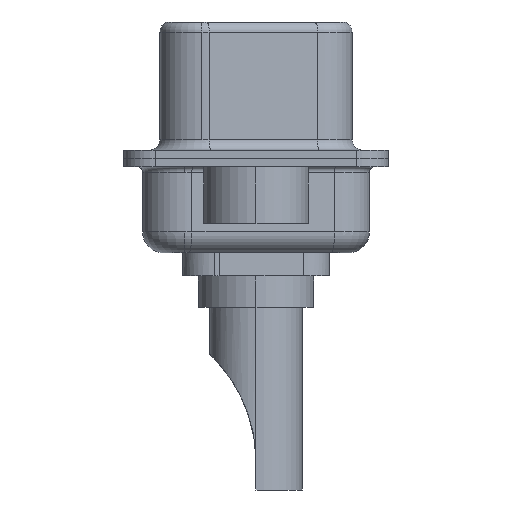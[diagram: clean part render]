
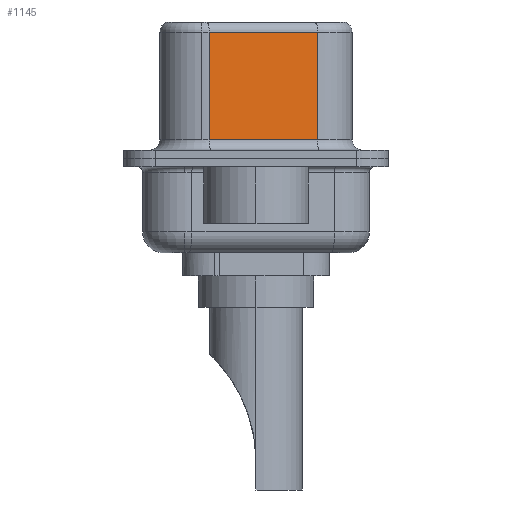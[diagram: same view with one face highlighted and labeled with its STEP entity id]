
A CAD part, left-side view. The second image highlights one B-rep face of the part: STEP entity #1145.
In plain terms, the highlighted planar face has unit normal (-0.985, -0.174, 0).
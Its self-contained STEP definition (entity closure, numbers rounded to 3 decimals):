
#921 = ORIENTED_EDGE ( 'NONE', *, *, #18159, .F. ) ;
#1145 = ADVANCED_FACE ( 'NONE', ( #7313 ), #12978, .F. ) ;
#1461 = CARTESIAN_POINT ( 'NONE',  ( 4.585, -2.927, 0.9 ) ) ;
#3293 = VERTEX_POINT ( 'NONE', #5164 ) ;
#3413 = VERTEX_POINT ( 'NONE', #20623 ) ;
#5068 = LINE ( 'NONE', #6559, #18393 ) ;
#5164 = CARTESIAN_POINT ( 'NONE',  ( 3.675, 2.233, 6.02 ) ) ;
#5823 = ORIENTED_EDGE ( 'NONE', *, *, #14037, .T. ) ;
#6559 = CARTESIAN_POINT ( 'NONE',  ( 4.585, -2.927, 0.9 ) ) ;
#7313 = FACE_OUTER_BOUND ( 'NONE', #21106, .T. ) ;
#7506 = DIRECTION ( 'NONE',  ( -0.174, 0.985, 0. ) ) ;
#8138 = VECTOR ( 'NONE', #14675, 1000. ) ;
#8716 = VECTOR ( 'NONE', #13194, 1000. ) ;
#10088 = ORIENTED_EDGE ( 'NONE', *, *, #10400, .T. ) ;
#10400 = EDGE_CURVE ( 'NONE', #3293, #3413, #13261, .T. ) ;
#10578 = ORIENTED_EDGE ( 'NONE', *, *, #11546, .T. ) ;
#11383 = CARTESIAN_POINT ( 'NONE',  ( 3.675, 2.233, 6.52 ) ) ;
#11546 = EDGE_CURVE ( 'NONE', #21036, #3293, #22047, .T. ) ;
#12978 = PLANE ( 'NONE',  #22401 ) ;
#13174 = CARTESIAN_POINT ( 'NONE',  ( 4.585, -2.927, 6.52 ) ) ;
#13194 = DIRECTION ( 'NONE',  ( 0., 0., -1. ) ) ;
#13261 = LINE ( 'NONE', #11383, #8716 ) ;
#14037 = EDGE_CURVE ( 'NONE', #3413, #22305, #5068, .T. ) ;
#14675 = DIRECTION ( 'NONE',  ( -0.174, 0.985, 0. ) ) ;
#14944 = DIRECTION ( 'NONE',  ( 0., 0., -1. ) ) ;
#15862 = DIRECTION ( 'NONE',  ( 0.985, 0.174, 0. ) ) ;
#16145 = VECTOR ( 'NONE', #14944, 1000. ) ;
#16718 = LINE ( 'NONE', #13174, #16145 ) ;
#18159 = EDGE_CURVE ( 'NONE', #21036, #22305, #16718, .T. ) ;
#18300 = CARTESIAN_POINT ( 'NONE',  ( 4.585, -2.927, 6.02 ) ) ;
#18393 = VECTOR ( 'NONE', #18714, 1000. ) ;
#18714 = DIRECTION ( 'NONE',  ( 0.174, -0.985, 0. ) ) ;
#20042 = CARTESIAN_POINT ( 'NONE',  ( 4.585, -2.927, 6.02 ) ) ;
#20623 = CARTESIAN_POINT ( 'NONE',  ( 3.675, 2.233, 0.9 ) ) ;
#21036 = VERTEX_POINT ( 'NONE', #20042 ) ;
#21106 = EDGE_LOOP ( 'NONE', ( #921, #10578, #10088, #5823 ) ) ;
#22047 = LINE ( 'NONE', #18300, #8138 ) ;
#22073 = CARTESIAN_POINT ( 'NONE',  ( 4.585, -2.927, 6.52 ) ) ;
#22305 = VERTEX_POINT ( 'NONE', #1461 ) ;
#22401 = AXIS2_PLACEMENT_3D ( 'NONE', #22073, #15862, #7506 ) ;
